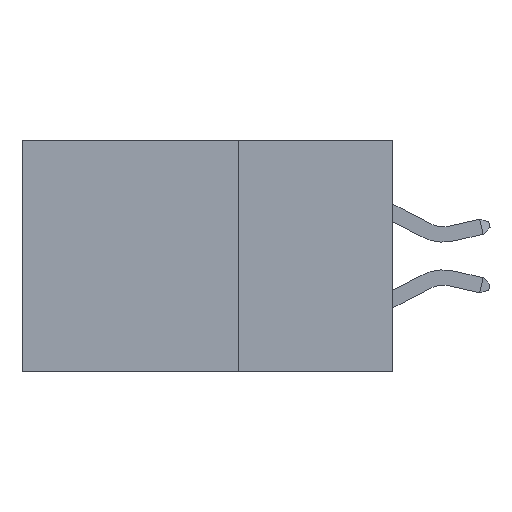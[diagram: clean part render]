
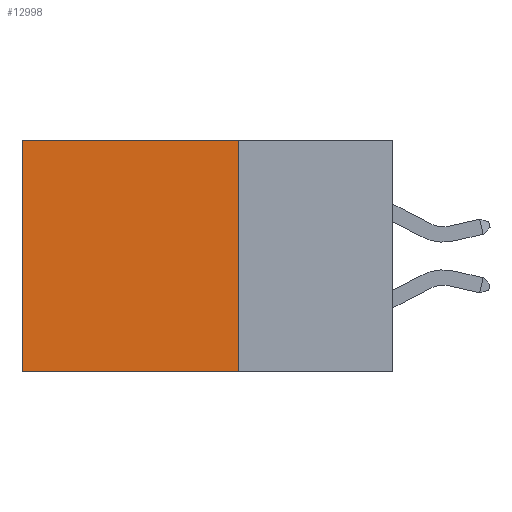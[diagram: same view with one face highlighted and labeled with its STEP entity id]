
A CAD part, left-side view. The second image highlights one B-rep face of the part: STEP entity #12998.
In plain terms, the highlighted planar face has unit normal (-1, 0, 0).
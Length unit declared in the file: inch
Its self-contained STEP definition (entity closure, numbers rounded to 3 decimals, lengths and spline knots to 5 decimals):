
#56 = DIRECTION ( 'NONE',  ( 0., 1., 0. ) ) ;
#754 = AXIS2_PLACEMENT_3D ( 'NONE', #18491, #15705, #6909 ) ;
#1208 = VERTEX_POINT ( 'NONE', #3597 ) ;
#1310 = EDGE_CURVE ( 'NONE', #1725, #7677, #13967, .T. ) ;
#1650 = EDGE_CURVE ( 'NONE', #1208, #16794, #5481, .T. ) ;
#1725 = VERTEX_POINT ( 'NONE', #6447 ) ;
#2287 = CARTESIAN_POINT ( 'NONE',  ( 0.2875, 0.25, -0.375 ) ) ;
#2829 = ORIENTED_EDGE ( 'NONE', *, *, #1650, .F. ) ;
#3132 = CARTESIAN_POINT ( 'NONE',  ( 0.2875, 0.6, 0. ) ) ;
#3597 = CARTESIAN_POINT ( 'NONE',  ( 0.2875, 0.25, -0.375 ) ) ;
#4428 = CARTESIAN_POINT ( 'NONE',  ( 0.2875, 0.25, 0. ) ) ;
#4555 = VECTOR ( 'NONE', #17879, 39.37008 ) ;
#5250 = EDGE_CURVE ( 'NONE', #1725, #1208, #15752, .T. ) ;
#5481 = LINE ( 'NONE', #6190, #4555 ) ;
#6190 = CARTESIAN_POINT ( 'NONE',  ( 0.2875, 0.25, -0.375 ) ) ;
#6447 = CARTESIAN_POINT ( 'NONE',  ( 0.2875, 0.25, 0. ) ) ;
#6480 = CARTESIAN_POINT ( 'NONE',  ( 0.2875, 0.6, -0.375 ) ) ;
#6625 = FACE_OUTER_BOUND ( 'NONE', #7325, .T. ) ;
#6909 = DIRECTION ( 'NONE',  ( 0., 0., -1. ) ) ;
#7325 = EDGE_LOOP ( 'NONE', ( #13984, #2829, #13226, #15617 ) ) ;
#7677 = VERTEX_POINT ( 'NONE', #3132 ) ;
#8316 = DIRECTION ( 'NONE',  ( 0., 0., -1. ) ) ;
#8375 = LINE ( 'NONE', #6480, #8595 ) ;
#8595 = VECTOR ( 'NONE', #15185, 39.37008 ) ;
#9377 = VECTOR ( 'NONE', #56, 39.37008 ) ;
#12553 = PLANE ( 'NONE',  #754 ) ;
#12998 = ADVANCED_FACE ( 'NONE', ( #6625 ), #12553, .F. ) ;
#13226 = ORIENTED_EDGE ( 'NONE', *, *, #5250, .F. ) ;
#13967 = LINE ( 'NONE', #4428, #9377 ) ;
#13984 = ORIENTED_EDGE ( 'NONE', *, *, #14735, .T. ) ;
#14357 = VECTOR ( 'NONE', #8316, 39.37008 ) ;
#14735 = EDGE_CURVE ( 'NONE', #7677, #16794, #8375, .T. ) ;
#15185 = DIRECTION ( 'NONE',  ( 0., 0., -1. ) ) ;
#15617 = ORIENTED_EDGE ( 'NONE', *, *, #1310, .T. ) ;
#15705 = DIRECTION ( 'NONE',  ( 1., 0., 0. ) ) ;
#15752 = LINE ( 'NONE', #2287, #14357 ) ;
#16794 = VERTEX_POINT ( 'NONE', #17152 ) ;
#17152 = CARTESIAN_POINT ( 'NONE',  ( 0.2875, 0.6, -0.375 ) ) ;
#17879 = DIRECTION ( 'NONE',  ( 0., 1., 0. ) ) ;
#18491 = CARTESIAN_POINT ( 'NONE',  ( 0.2875, 0.25, -0.375 ) ) ;
